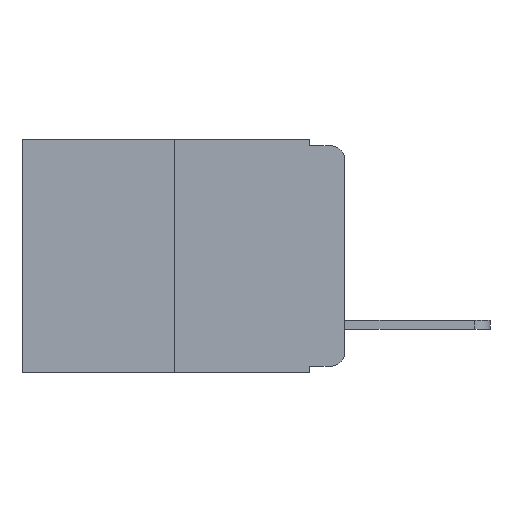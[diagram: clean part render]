
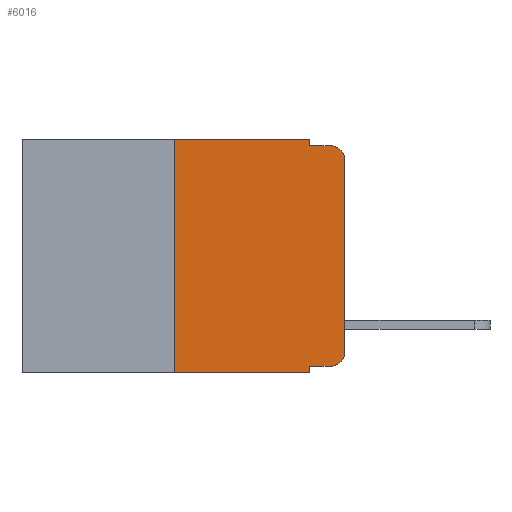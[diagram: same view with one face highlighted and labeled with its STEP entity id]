
A CAD part, left-side view. The second image highlights one B-rep face of the part: STEP entity #6016.
In plain terms, the highlighted planar face has unit normal (-1, 0, 0).
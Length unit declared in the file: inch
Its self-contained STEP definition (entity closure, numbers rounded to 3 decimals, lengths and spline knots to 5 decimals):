
#49 = VECTOR ( 'NONE', #4903, 39.37008 ) ;
#265 = LINE ( 'NONE', #12458, #10669 ) ;
#463 = VERTEX_POINT ( 'NONE', #3389 ) ;
#492 = VERTEX_POINT ( 'NONE', #11484 ) ;
#742 = CARTESIAN_POINT ( 'NONE',  ( 0., 0., -0.03 ) ) ;
#749 = LINE ( 'NONE', #5195, #8630 ) ;
#800 = VERTEX_POINT ( 'NONE', #12655 ) ;
#864 = EDGE_CURVE ( 'NONE', #12123, #5931, #3168, .T. ) ;
#911 = CARTESIAN_POINT ( 'NONE',  ( 0., 0.02, -0.03 ) ) ;
#1311 = ORIENTED_EDGE ( 'NONE', *, *, #2339, .F. ) ;
#1541 = EDGE_CURVE ( 'NONE', #463, #12123, #11810, .T. ) ;
#1928 = ORIENTED_EDGE ( 'NONE', *, *, #1955, .F. ) ;
#1955 = EDGE_CURVE ( 'NONE', #5931, #9617, #265, .T. ) ;
#1984 = LINE ( 'NONE', #7108, #7142 ) ;
#2118 = DIRECTION ( 'NONE',  ( 0., -1., 0. ) ) ;
#2187 = CARTESIAN_POINT ( 'NONE',  ( 0., 0.02, -0.313 ) ) ;
#2339 = EDGE_CURVE ( 'NONE', #9617, #9003, #10480, .T. ) ;
#2821 = VERTEX_POINT ( 'NONE', #7675 ) ;
#2846 = ORIENTED_EDGE ( 'NONE', *, *, #3263, .T. ) ;
#2954 = CARTESIAN_POINT ( 'NONE',  ( 0., 0.473, -0.343 ) ) ;
#3079 = EDGE_LOOP ( 'NONE', ( #7218, #2846, #1311, #1928, #9907, #8785, #8145, #11669, #11572, #4325 ) ) ;
#3168 = LINE ( 'NONE', #6403, #8119 ) ;
#3263 = EDGE_CURVE ( 'NONE', #5226, #9003, #7007, .T. ) ;
#3305 = DIRECTION ( 'NONE',  ( 0., 0., -1. ) ) ;
#3351 = EDGE_CURVE ( 'NONE', #11214, #5226, #749, .T. ) ;
#3389 = CARTESIAN_POINT ( 'NONE',  ( 0., 0.25, -0.343 ) ) ;
#3433 = DIRECTION ( 'NONE',  ( 0., 0., 1. ) ) ;
#3473 = DIRECTION ( 'NONE',  ( 0., 0., 1. ) ) ;
#3682 = CARTESIAN_POINT ( 'NONE',  ( 0., 0.051, -0.01 ) ) ;
#4035 = DIRECTION ( 'NONE',  ( 0., -1., 0. ) ) ;
#4277 = CARTESIAN_POINT ( 'NONE',  ( 0., 0., -0.313 ) ) ;
#4325 = ORIENTED_EDGE ( 'NONE', *, *, #11940, .T. ) ;
#4903 = DIRECTION ( 'NONE',  ( 0., -1., 0. ) ) ;
#5195 = CARTESIAN_POINT ( 'NONE',  ( 0., 0., 0. ) ) ;
#5226 = VERTEX_POINT ( 'NONE', #742 ) ;
#5297 = CARTESIAN_POINT ( 'NONE',  ( 0., 0.473, 0. ) ) ;
#5346 = DIRECTION ( 'NONE',  ( 1., 0., 0. ) ) ;
#5931 = VERTEX_POINT ( 'NONE', #7974 ) ;
#6016 = ADVANCED_FACE ( 'NONE', ( #10396 ), #10088, .F. ) ;
#6096 = CARTESIAN_POINT ( 'NONE',  ( 0., 0.051, 0. ) ) ;
#6323 = EDGE_CURVE ( 'NONE', #463, #2821, #12676, .T. ) ;
#6403 = CARTESIAN_POINT ( 'NONE',  ( 0., 0.473, 0. ) ) ;
#6423 = CIRCLE ( 'NONE', #11076, 0.02 ) ;
#7007 = CIRCLE ( 'NONE', #8653, 0.02 ) ;
#7108 = CARTESIAN_POINT ( 'NONE',  ( 0., 0.051, -0.333 ) ) ;
#7142 = VECTOR ( 'NONE', #8050, 39.37008 ) ;
#7218 = ORIENTED_EDGE ( 'NONE', *, *, #3351, .T. ) ;
#7535 = CARTESIAN_POINT ( 'NONE',  ( 0., 0.25, 0. ) ) ;
#7675 = CARTESIAN_POINT ( 'NONE',  ( 0., 0.051, -0.343 ) ) ;
#7953 = VECTOR ( 'NONE', #4035, 39.37008 ) ;
#7974 = CARTESIAN_POINT ( 'NONE',  ( 0., 0.051, 0. ) ) ;
#8018 = LINE ( 'NONE', #6096, #11724 ) ;
#8050 = DIRECTION ( 'NONE',  ( 0., -1., 0. ) ) ;
#8119 = VECTOR ( 'NONE', #2118, 39.37008 ) ;
#8145 = ORIENTED_EDGE ( 'NONE', *, *, #6323, .T. ) ;
#8413 = EDGE_CURVE ( 'NONE', #800, #2821, #8018, .T. ) ;
#8458 = CARTESIAN_POINT ( 'NONE',  ( 0., 0.25, 0. ) ) ;
#8630 = VECTOR ( 'NONE', #3433, 39.37008 ) ;
#8653 = AXIS2_PLACEMENT_3D ( 'NONE', #911, #9214, #9189 ) ;
#8785 = ORIENTED_EDGE ( 'NONE', *, *, #1541, .F. ) ;
#9003 = VERTEX_POINT ( 'NONE', #11297 ) ;
#9189 = DIRECTION ( 'NONE',  ( 0., 0., -1. ) ) ;
#9199 = DIRECTION ( 'NONE',  ( -1., 0., 0. ) ) ;
#9214 = DIRECTION ( 'NONE',  ( -1., 0., 0. ) ) ;
#9360 = CARTESIAN_POINT ( 'NONE',  ( 0., 0.051, -0.01 ) ) ;
#9482 = AXIS2_PLACEMENT_3D ( 'NONE', #5297, #5346, #11872 ) ;
#9617 = VERTEX_POINT ( 'NONE', #9360 ) ;
#9907 = ORIENTED_EDGE ( 'NONE', *, *, #864, .F. ) ;
#9930 = DIRECTION ( 'NONE',  ( 0., 0., -1. ) ) ;
#10088 = PLANE ( 'NONE',  #9482 ) ;
#10396 = FACE_OUTER_BOUND ( 'NONE', #3079, .T. ) ;
#10469 = DIRECTION ( 'NONE',  ( 0., 0., -1. ) ) ;
#10480 = LINE ( 'NONE', #3682, #49 ) ;
#10669 = VECTOR ( 'NONE', #10469, 39.37008 ) ;
#11076 = AXIS2_PLACEMENT_3D ( 'NONE', #2187, #9199, #3305 ) ;
#11214 = VERTEX_POINT ( 'NONE', #4277 ) ;
#11252 = VECTOR ( 'NONE', #3473, 39.37008 ) ;
#11297 = CARTESIAN_POINT ( 'NONE',  ( 0., 0.02, -0.01 ) ) ;
#11484 = CARTESIAN_POINT ( 'NONE',  ( 0., 0.02, -0.333 ) ) ;
#11572 = ORIENTED_EDGE ( 'NONE', *, *, #12709, .T. ) ;
#11669 = ORIENTED_EDGE ( 'NONE', *, *, #8413, .F. ) ;
#11724 = VECTOR ( 'NONE', #9930, 39.37008 ) ;
#11810 = LINE ( 'NONE', #8458, #11252 ) ;
#11872 = DIRECTION ( 'NONE',  ( 0., 0., -1. ) ) ;
#11940 = EDGE_CURVE ( 'NONE', #492, #11214, #6423, .T. ) ;
#12123 = VERTEX_POINT ( 'NONE', #7535 ) ;
#12458 = CARTESIAN_POINT ( 'NONE',  ( 0., 0.051, 0. ) ) ;
#12655 = CARTESIAN_POINT ( 'NONE',  ( 0., 0.051, -0.333 ) ) ;
#12676 = LINE ( 'NONE', #2954, #7953 ) ;
#12709 = EDGE_CURVE ( 'NONE', #800, #492, #1984, .T. ) ;
